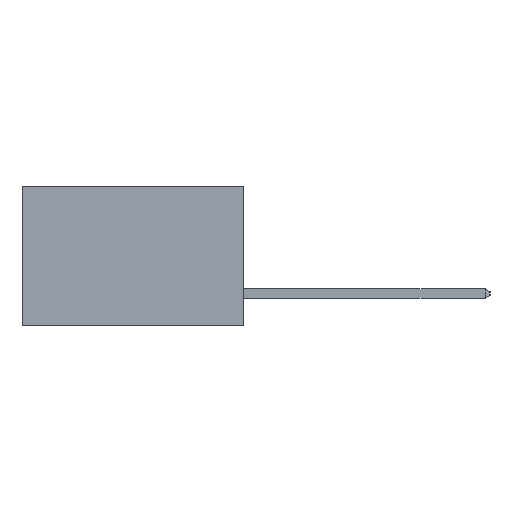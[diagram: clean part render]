
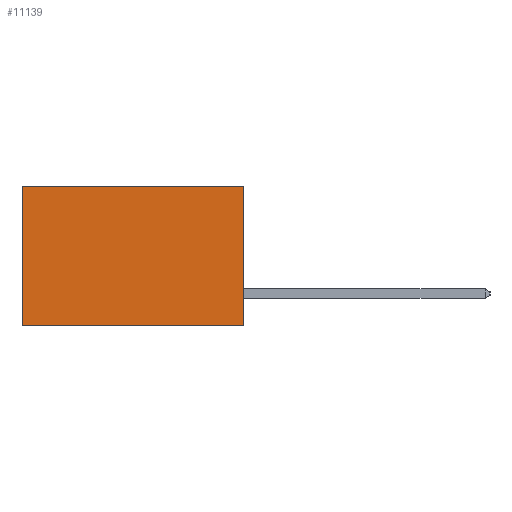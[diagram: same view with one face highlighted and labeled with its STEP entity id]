
A CAD part, left-side view. The second image highlights one B-rep face of the part: STEP entity #11139.
In plain terms, the highlighted planar face has unit normal (-1, 0, 0).
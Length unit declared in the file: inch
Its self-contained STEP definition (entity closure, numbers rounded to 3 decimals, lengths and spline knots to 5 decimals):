
#302 = VECTOR ( 'NONE', #2598, 39.37008 ) ;
#1356 = DIRECTION ( 'NONE',  ( 1., 0., 0. ) ) ;
#1987 = EDGE_CURVE ( 'NONE', #8316, #5314, #15832, .T. ) ;
#2481 = CARTESIAN_POINT ( 'NONE',  ( 0.277, 0.59, -0.37 ) ) ;
#2598 = DIRECTION ( 'NONE',  ( 0., 0., -1. ) ) ;
#2937 = VERTEX_POINT ( 'NONE', #3871 ) ;
#3340 = EDGE_CURVE ( 'NONE', #5314, #21673, #20692, .T. ) ;
#3871 = CARTESIAN_POINT ( 'NONE',  ( 0.277, 0.59, 0. ) ) ;
#5314 = VERTEX_POINT ( 'NONE', #21830 ) ;
#6225 = DIRECTION ( 'NONE',  ( 0., 1., 0. ) ) ;
#6684 = CARTESIAN_POINT ( 'NONE',  ( 0.277, 0., 0. ) ) ;
#6836 = VECTOR ( 'NONE', #6225, 39.37008 ) ;
#8060 = CARTESIAN_POINT ( 'NONE',  ( 0.277, 0., -0.37 ) ) ;
#8316 = VERTEX_POINT ( 'NONE', #15241 ) ;
#10122 = VECTOR ( 'NONE', #10614, 39.37008 ) ;
#10614 = DIRECTION ( 'NONE',  ( 0., 1., 0. ) ) ;
#11139 = ADVANCED_FACE ( 'NONE', ( #20022 ), #24237, .F. ) ;
#11156 = CARTESIAN_POINT ( 'NONE',  ( 0.277, 0., -0.37 ) ) ;
#12518 = VECTOR ( 'NONE', #19670, 39.37008 ) ;
#12742 = AXIS2_PLACEMENT_3D ( 'NONE', #11156, #1356, #14955 ) ;
#13187 = CARTESIAN_POINT ( 'NONE',  ( 0.277, 0.59, -0.37 ) ) ;
#14513 = ORIENTED_EDGE ( 'NONE', *, *, #1987, .F. ) ;
#14936 = ORIENTED_EDGE ( 'NONE', *, *, #16426, .T. ) ;
#14955 = DIRECTION ( 'NONE',  ( 0., 0., -1. ) ) ;
#15153 = LINE ( 'NONE', #6684, #10122 ) ;
#15241 = CARTESIAN_POINT ( 'NONE',  ( 0.277, 0., 0. ) ) ;
#15832 = LINE ( 'NONE', #8060, #302 ) ;
#15984 = ORIENTED_EDGE ( 'NONE', *, *, #16341, .T. ) ;
#16341 = EDGE_CURVE ( 'NONE', #2937, #21673, #22428, .T. ) ;
#16426 = EDGE_CURVE ( 'NONE', #8316, #2937, #15153, .T. ) ;
#17448 = ORIENTED_EDGE ( 'NONE', *, *, #3340, .F. ) ;
#18136 = EDGE_LOOP ( 'NONE', ( #15984, #17448, #14513, #14936 ) ) ;
#19160 = CARTESIAN_POINT ( 'NONE',  ( 0.277, 0., -0.37 ) ) ;
#19670 = DIRECTION ( 'NONE',  ( 0., 0., -1. ) ) ;
#20022 = FACE_OUTER_BOUND ( 'NONE', #18136, .T. ) ;
#20692 = LINE ( 'NONE', #19160, #6836 ) ;
#21673 = VERTEX_POINT ( 'NONE', #13187 ) ;
#21830 = CARTESIAN_POINT ( 'NONE',  ( 0.277, 0., -0.37 ) ) ;
#22428 = LINE ( 'NONE', #2481, #12518 ) ;
#24237 = PLANE ( 'NONE',  #12742 ) ;
